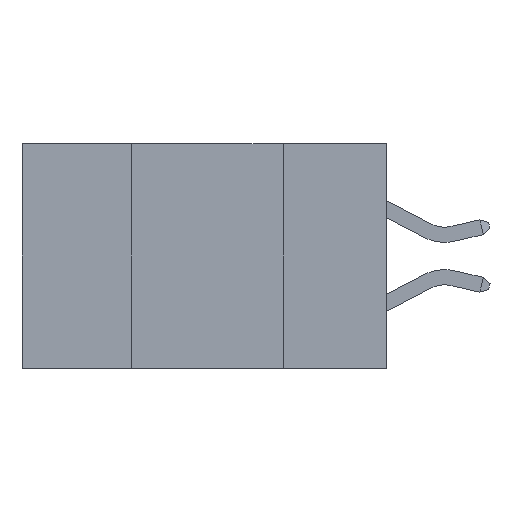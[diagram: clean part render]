
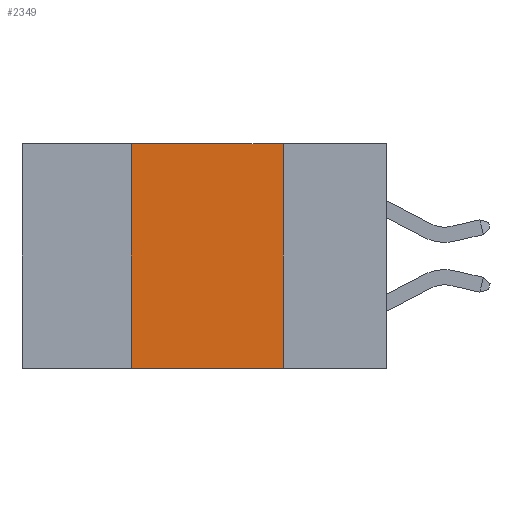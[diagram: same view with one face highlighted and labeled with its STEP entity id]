
A CAD part, left-side view. The second image highlights one B-rep face of the part: STEP entity #2349.
In plain terms, the highlighted planar face has unit normal (-1, 0, 0).
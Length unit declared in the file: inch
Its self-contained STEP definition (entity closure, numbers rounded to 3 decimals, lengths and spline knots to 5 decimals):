
#808 = EDGE_CURVE ( 'NONE', #23170, #14570, #1834, .T. ) ;
#1834 = LINE ( 'NONE', #11503, #7619 ) ;
#2349 = ADVANCED_FACE ( 'NONE', ( #19393 ), #21725, .F. ) ;
#3195 = AXIS2_PLACEMENT_3D ( 'NONE', #12167, #21886, #17718 ) ;
#3793 = VECTOR ( 'NONE', #19428, 39.37008 ) ;
#4275 = CARTESIAN_POINT ( 'NONE',  ( 0., 0.17, -0.37 ) ) ;
#7139 = EDGE_CURVE ( 'NONE', #23170, #20196, #11752, .T. ) ;
#7363 = ORIENTED_EDGE ( 'NONE', *, *, #18542, .F. ) ;
#7377 = DIRECTION ( 'NONE',  ( 0., 0., 1. ) ) ;
#7619 = VECTOR ( 'NONE', #7377, 39.37008 ) ;
#7925 = CARTESIAN_POINT ( 'NONE',  ( 0., 0.17, 0. ) ) ;
#8997 = DIRECTION ( 'NONE',  ( 0., -1., 0. ) ) ;
#11213 = EDGE_CURVE ( 'NONE', #12932, #20196, #19095, .T. ) ;
#11503 = CARTESIAN_POINT ( 'NONE',  ( 0., 0.42, 0. ) ) ;
#11752 = LINE ( 'NONE', #15120, #16679 ) ;
#12167 = CARTESIAN_POINT ( 'NONE',  ( 0., 0.6, 0. ) ) ;
#12932 = VERTEX_POINT ( 'NONE', #23837 ) ;
#14387 = ORIENTED_EDGE ( 'NONE', *, *, #7139, .T. ) ;
#14512 = CARTESIAN_POINT ( 'NONE',  ( 0., 0.42, 0. ) ) ;
#14570 = VERTEX_POINT ( 'NONE', #14512 ) ;
#15120 = CARTESIAN_POINT ( 'NONE',  ( 0., 0.6, -0.37 ) ) ;
#16007 = DIRECTION ( 'NONE',  ( 0., 0., -1. ) ) ;
#16679 = VECTOR ( 'NONE', #8997, 39.37008 ) ;
#16800 = ORIENTED_EDGE ( 'NONE', *, *, #11213, .F. ) ;
#17491 = CARTESIAN_POINT ( 'NONE',  ( 0., 0.6, 0. ) ) ;
#17718 = DIRECTION ( 'NONE',  ( 0., 0., -1. ) ) ;
#18542 = EDGE_CURVE ( 'NONE', #14570, #12932, #22941, .T. ) ;
#19095 = LINE ( 'NONE', #7925, #19391 ) ;
#19391 = VECTOR ( 'NONE', #16007, 39.37008 ) ;
#19393 = FACE_OUTER_BOUND ( 'NONE', #20079, .T. ) ;
#19428 = DIRECTION ( 'NONE',  ( 0., -1., 0. ) ) ;
#20079 = EDGE_LOOP ( 'NONE', ( #16800, #7363, #23445, #14387 ) ) ;
#20196 = VERTEX_POINT ( 'NONE', #4275 ) ;
#21725 = PLANE ( 'NONE',  #3195 ) ;
#21886 = DIRECTION ( 'NONE',  ( 1., 0., 0. ) ) ;
#22941 = LINE ( 'NONE', #17491, #3793 ) ;
#23170 = VERTEX_POINT ( 'NONE', #24947 ) ;
#23445 = ORIENTED_EDGE ( 'NONE', *, *, #808, .F. ) ;
#23837 = CARTESIAN_POINT ( 'NONE',  ( 0., 0.17, 0. ) ) ;
#24947 = CARTESIAN_POINT ( 'NONE',  ( 0., 0.42, -0.37 ) ) ;
